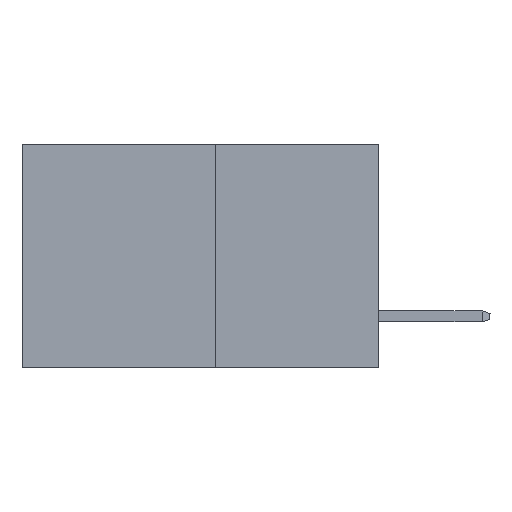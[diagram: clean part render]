
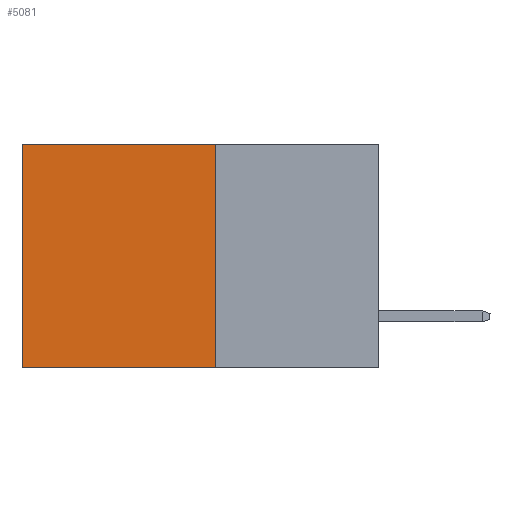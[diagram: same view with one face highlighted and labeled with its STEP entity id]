
A CAD part, left-side view. The second image highlights one B-rep face of the part: STEP entity #5081.
In plain terms, the highlighted planar face has unit normal (-1, 0, 0).
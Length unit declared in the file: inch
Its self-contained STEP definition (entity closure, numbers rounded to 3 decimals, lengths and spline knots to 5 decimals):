
#828 = ORIENTED_EDGE ( 'NONE', *, *, #4569, .F. ) ;
#1057 = ORIENTED_EDGE ( 'NONE', *, *, #3032, .F. ) ;
#1225 = DIRECTION ( 'NONE',  ( 0., 0., -1. ) ) ;
#1307 = LINE ( 'NONE', #5117, #7689 ) ;
#1890 = DIRECTION ( 'NONE',  ( 0., 0., -1. ) ) ;
#1922 = DIRECTION ( 'NONE',  ( 1., 0., 0. ) ) ;
#1930 = CARTESIAN_POINT ( 'NONE',  ( 0.277, 0.27, -0.37 ) ) ;
#2026 = PLANE ( 'NONE',  #9110 ) ;
#2513 = LINE ( 'NONE', #5839, #4622 ) ;
#2548 = CARTESIAN_POINT ( 'NONE',  ( 0.277, 0.27, -0.37 ) ) ;
#2574 = EDGE_LOOP ( 'NONE', ( #5400, #1057, #828, #9547 ) ) ;
#2596 = EDGE_CURVE ( 'NONE', #3215, #7768, #1307, .T. ) ;
#2794 = VERTEX_POINT ( 'NONE', #2548 ) ;
#3032 = EDGE_CURVE ( 'NONE', #2794, #5545, #8021, .T. ) ;
#3215 = VERTEX_POINT ( 'NONE', #6530 ) ;
#3645 = VECTOR ( 'NONE', #8720, 39.37008 ) ;
#3682 = FACE_OUTER_BOUND ( 'NONE', #2574, .T. ) ;
#3832 = VECTOR ( 'NONE', #4949, 39.37008 ) ;
#4108 = LINE ( 'NONE', #4996, #3832 ) ;
#4569 = EDGE_CURVE ( 'NONE', #3215, #2794, #4108, .T. ) ;
#4622 = VECTOR ( 'NONE', #1225, 39.37008 ) ;
#4949 = DIRECTION ( 'NONE',  ( 0., 0., -1. ) ) ;
#4996 = CARTESIAN_POINT ( 'NONE',  ( 0.277, 0.27, -0.37 ) ) ;
#5076 = DIRECTION ( 'NONE',  ( 0., 1., 0. ) ) ;
#5081 = ADVANCED_FACE ( 'NONE', ( #3682 ), #2026, .F. ) ;
#5117 = CARTESIAN_POINT ( 'NONE',  ( 0.277, 0.27, 0. ) ) ;
#5192 = EDGE_CURVE ( 'NONE', #7768, #5545, #2513, .T. ) ;
#5400 = ORIENTED_EDGE ( 'NONE', *, *, #5192, .T. ) ;
#5545 = VERTEX_POINT ( 'NONE', #9026 ) ;
#5839 = CARTESIAN_POINT ( 'NONE',  ( 0.277, 0.59, -0.37 ) ) ;
#6530 = CARTESIAN_POINT ( 'NONE',  ( 0.277, 0.27, 0. ) ) ;
#7550 = CARTESIAN_POINT ( 'NONE',  ( 0.277, 0.59, 0. ) ) ;
#7689 = VECTOR ( 'NONE', #5076, 39.37008 ) ;
#7768 = VERTEX_POINT ( 'NONE', #7550 ) ;
#8021 = LINE ( 'NONE', #8956, #3645 ) ;
#8720 = DIRECTION ( 'NONE',  ( 0., 1., 0. ) ) ;
#8956 = CARTESIAN_POINT ( 'NONE',  ( 0.277, 0.27, -0.37 ) ) ;
#9026 = CARTESIAN_POINT ( 'NONE',  ( 0.277, 0.59, -0.37 ) ) ;
#9110 = AXIS2_PLACEMENT_3D ( 'NONE', #1930, #1922, #1890 ) ;
#9547 = ORIENTED_EDGE ( 'NONE', *, *, #2596, .T. ) ;
